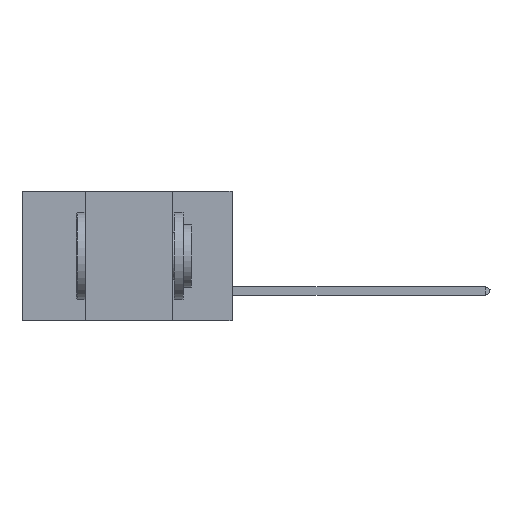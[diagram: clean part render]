
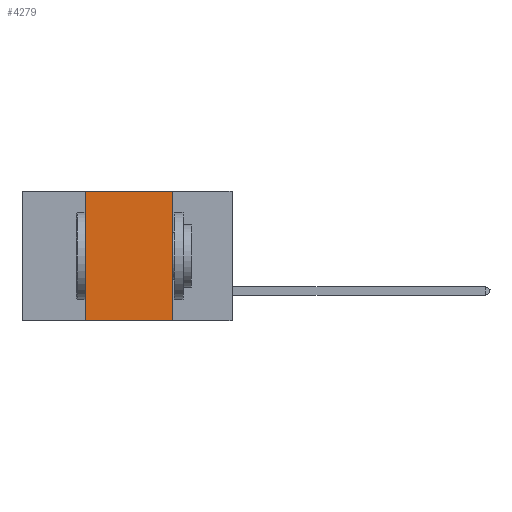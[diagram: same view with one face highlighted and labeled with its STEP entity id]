
A CAD part, left-side view. The second image highlights one B-rep face of the part: STEP entity #4279.
In plain terms, the highlighted planar face has unit normal (-1, 0, 0).
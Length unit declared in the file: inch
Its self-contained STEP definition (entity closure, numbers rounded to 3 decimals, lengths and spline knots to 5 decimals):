
#182 = ORIENTED_EDGE ( 'NONE', *, *, #1142, .F. ) ;
#1142 = EDGE_CURVE ( 'NONE', #7685, #18459, #8728, .T. ) ;
#1903 = VECTOR ( 'NONE', #14865, 39.37008 ) ;
#2685 = CARTESIAN_POINT ( 'NONE',  ( 0., 0.17, -0.37 ) ) ;
#3014 = FACE_OUTER_BOUND ( 'NONE', #14895, .T. ) ;
#3591 = CARTESIAN_POINT ( 'NONE',  ( 0., 0.17, 0. ) ) ;
#4093 = VECTOR ( 'NONE', #4456, 39.37008 ) ;
#4279 = ADVANCED_FACE ( 'NONE', ( #3014 ), #12172, .F. ) ;
#4456 = DIRECTION ( 'NONE',  ( 0., -1., 0. ) ) ;
#6394 = CARTESIAN_POINT ( 'NONE',  ( 0., 0.6, -0.37 ) ) ;
#6417 = DIRECTION ( 'NONE',  ( 0., 0., 1. ) ) ;
#6930 = ORIENTED_EDGE ( 'NONE', *, *, #12838, .F. ) ;
#7305 = VECTOR ( 'NONE', #16882, 39.37008 ) ;
#7685 = VERTEX_POINT ( 'NONE', #13646 ) ;
#7816 = EDGE_CURVE ( 'NONE', #10512, #12139, #11326, .T. ) ;
#8728 = LINE ( 'NONE', #17905, #4093 ) ;
#9559 = EDGE_CURVE ( 'NONE', #18459, #12139, #17126, .T. ) ;
#9806 = CARTESIAN_POINT ( 'NONE',  ( 0., 0.6, 0. ) ) ;
#10512 = VERTEX_POINT ( 'NONE', #18019 ) ;
#10805 = AXIS2_PLACEMENT_3D ( 'NONE', #9806, #17297, #13995 ) ;
#11326 = LINE ( 'NONE', #6394, #7305 ) ;
#12139 = VERTEX_POINT ( 'NONE', #2685 ) ;
#12172 = PLANE ( 'NONE',  #10805 ) ;
#12838 = EDGE_CURVE ( 'NONE', #10512, #7685, #18267, .T. ) ;
#13309 = ORIENTED_EDGE ( 'NONE', *, *, #7816, .T. ) ;
#13310 = VECTOR ( 'NONE', #6417, 39.37008 ) ;
#13646 = CARTESIAN_POINT ( 'NONE',  ( 0., 0.42, 0. ) ) ;
#13995 = DIRECTION ( 'NONE',  ( 0., 0., -1. ) ) ;
#14269 = ORIENTED_EDGE ( 'NONE', *, *, #9559, .F. ) ;
#14865 = DIRECTION ( 'NONE',  ( 0., 0., -1. ) ) ;
#14895 = EDGE_LOOP ( 'NONE', ( #14269, #182, #6930, #13309 ) ) ;
#16882 = DIRECTION ( 'NONE',  ( 0., -1., 0. ) ) ;
#17126 = LINE ( 'NONE', #18021, #1903 ) ;
#17297 = DIRECTION ( 'NONE',  ( 1., 0., 0. ) ) ;
#17905 = CARTESIAN_POINT ( 'NONE',  ( 0., 0.6, 0. ) ) ;
#18019 = CARTESIAN_POINT ( 'NONE',  ( 0., 0.42, -0.37 ) ) ;
#18021 = CARTESIAN_POINT ( 'NONE',  ( 0., 0.17, 0. ) ) ;
#18267 = LINE ( 'NONE', #19419, #13310 ) ;
#18459 = VERTEX_POINT ( 'NONE', #3591 ) ;
#19419 = CARTESIAN_POINT ( 'NONE',  ( 0., 0.42, 0. ) ) ;
